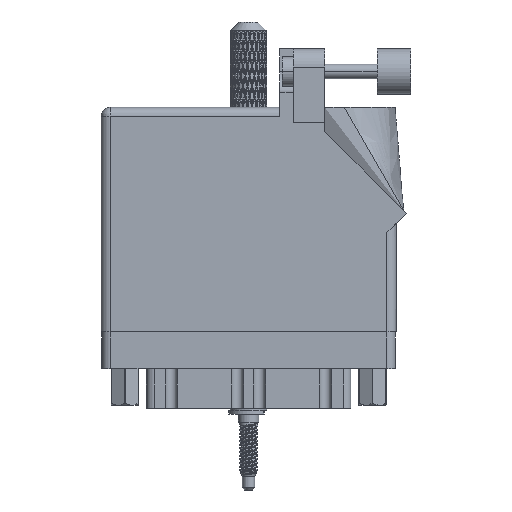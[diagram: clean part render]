
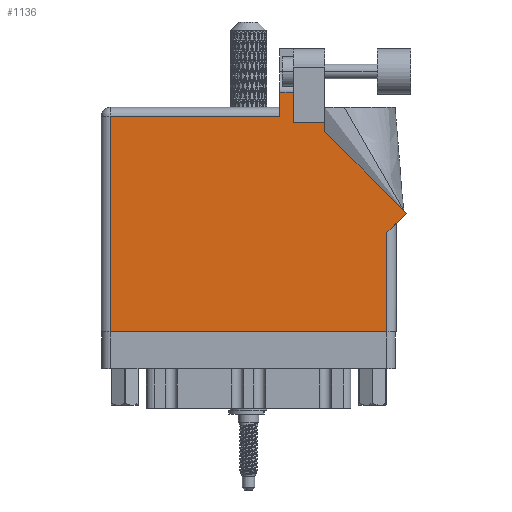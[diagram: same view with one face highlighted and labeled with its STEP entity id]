
A CAD part, front view. The second image highlights one B-rep face of the part: STEP entity #1136.
In plain terms, the highlighted face is planar.
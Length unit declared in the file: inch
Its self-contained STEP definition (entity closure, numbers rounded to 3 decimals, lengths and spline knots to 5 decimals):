
#1136 = ADVANCED_FACE ( 'NONE', ( #10595 ), #45646, .F. ) ;
#2997 = LINE ( 'NONE', #74816, #9502 ) ;
#4822 = LINE ( 'NONE', #14010, #57075 ) ;
#6854 = LINE ( 'NONE', #15484, #92922 ) ;
#8082 = VERTEX_POINT ( 'NONE', #25683 ) ;
#8295 = CARTESIAN_POINT ( 'NONE',  ( 1.948, 0., 0. ) ) ;
#8691 = VERTEX_POINT ( 'NONE', #42539 ) ;
#9327 = EDGE_CURVE ( 'NONE', #81317, #76900, #113542, .T. ) ;
#9394 = AXIS2_PLACEMENT_3D ( 'NONE', #80768, #61779, #37022 ) ;
#9502 = VECTOR ( 'NONE', #55290, 39.37008 ) ;
#9596 = ORIENTED_EDGE ( 'NONE', *, *, #113072, .T. ) ;
#10595 = FACE_OUTER_BOUND ( 'NONE', #31762, .T. ) ;
#11411 = EDGE_CURVE ( 'NONE', #18985, #8082, #17334, .T. ) ;
#14010 = CARTESIAN_POINT ( 'NONE',  ( 1.217, 1.53, 0. ) ) ;
#15283 = VECTOR ( 'NONE', #52614, 39.37008 ) ;
#15484 = CARTESIAN_POINT ( 'NONE',  ( 0., 1.468, 0. ) ) ;
#16804 = VECTOR ( 'NONE', #99911, 39.37008 ) ;
#17334 = LINE ( 'NONE', #52379, #65106 ) ;
#18728 = CARTESIAN_POINT ( 'NONE',  ( 2.08071, 0.80771, 0. ) ) ;
#18985 = VERTEX_POINT ( 'NONE', #39237 ) ;
#19264 = VECTOR ( 'NONE', #32398, 39.37008 ) ;
#20543 = CARTESIAN_POINT ( 'NONE',  ( 2.08071, 0.80771, 0. ) ) ;
#23062 = CARTESIAN_POINT ( 'NONE',  ( 1.311, 1.43, 0. ) ) ;
#23773 = VERTEX_POINT ( 'NONE', #82918 ) ;
#25299 = DIRECTION ( 'NONE',  ( 0., 1., 0. ) ) ;
#25683 = CARTESIAN_POINT ( 'NONE',  ( 1.311, 1.43, 0. ) ) ;
#27640 = VERTEX_POINT ( 'NONE', #107854 ) ;
#28287 = DIRECTION ( 'NONE',  ( 0., 1., 0. ) ) ;
#28886 = ORIENTED_EDGE ( 'NONE', *, *, #92803, .T. ) ;
#29039 = ORIENTED_EDGE ( 'NONE', *, *, #9327, .T. ) ;
#30234 = VECTOR ( 'NONE', #28287, 39.37008 ) ;
#31762 = EDGE_LOOP ( 'NONE', ( #52527, #9596, #28886, #35007, #96302, #73149, #81887, #29039, #71858, #47475, #35732 ) ) ;
#32072 = CARTESIAN_POINT ( 'NONE',  ( 1.217, 1.6315, 0. ) ) ;
#32131 = VERTEX_POINT ( 'NONE', #8295 ) ;
#32398 = DIRECTION ( 'NONE',  ( -0.707, 0.707, 0. ) ) ;
#34761 = DIRECTION ( 'NONE',  ( 0.707, 0.707, 0. ) ) ;
#34964 = EDGE_CURVE ( 'NONE', #32131, #81317, #70885, .T. ) ;
#35007 = ORIENTED_EDGE ( 'NONE', *, *, #108869, .T. ) ;
#35732 = ORIENTED_EDGE ( 'NONE', *, *, #11411, .T. ) ;
#37022 = DIRECTION ( 'NONE',  ( -1., 0., 0. ) ) ;
#39237 = CARTESIAN_POINT ( 'NONE',  ( 1.524, 1.43, 0. ) ) ;
#39376 = EDGE_CURVE ( 'NONE', #27640, #8691, #41122, .T. ) ;
#40375 = VECTOR ( 'NONE', #34761, 39.37008 ) ;
#40586 = VERTEX_POINT ( 'NONE', #61875 ) ;
#41122 = LINE ( 'NONE', #67587, #50276 ) ;
#42539 = CARTESIAN_POINT ( 'NONE',  ( 0.062, 0., 0. ) ) ;
#42853 = CARTESIAN_POINT ( 'NONE',  ( 2.01, 0.737, 0. ) ) ;
#43840 = EDGE_CURVE ( 'NONE', #23773, #18985, #87727, .T. ) ;
#45582 = CARTESIAN_POINT ( 'NONE',  ( 1.311, 1.6315, 0. ) ) ;
#45646 = PLANE ( 'NONE',  #9394 ) ;
#47475 = ORIENTED_EDGE ( 'NONE', *, *, #43840, .T. ) ;
#50276 = VECTOR ( 'NONE', #57240, 39.37008 ) ;
#50436 = VERTEX_POINT ( 'NONE', #32072 ) ;
#52379 = CARTESIAN_POINT ( 'NONE',  ( 1.524, 1.43, 0. ) ) ;
#52527 = ORIENTED_EDGE ( 'NONE', *, *, #66030, .T. ) ;
#52614 = DIRECTION ( 'NONE',  ( 0., 1., 0. ) ) ;
#52936 = DIRECTION ( 'NONE',  ( -1., 0., 0. ) ) ;
#53901 = VERTEX_POINT ( 'NONE', #45582 ) ;
#55290 = DIRECTION ( 'NONE',  ( 1., 0., 0. ) ) ;
#57075 = VECTOR ( 'NONE', #99722, 39.37008 ) ;
#57240 = DIRECTION ( 'NONE',  ( 0., -1., 0. ) ) ;
#61779 = DIRECTION ( 'NONE',  ( 0., 0., -1. ) ) ;
#61875 = CARTESIAN_POINT ( 'NONE',  ( 1.217, 1.468, 0. ) ) ;
#63960 = EDGE_CURVE ( 'NONE', #8691, #32131, #2997, .T. ) ;
#64825 = LINE ( 'NONE', #89596, #16804 ) ;
#65106 = VECTOR ( 'NONE', #52936, 39.37008 ) ;
#66030 = EDGE_CURVE ( 'NONE', #8082, #53901, #76524, .T. ) ;
#67258 = DIRECTION ( 'NONE',  ( -1., 0., 0. ) ) ;
#67587 = CARTESIAN_POINT ( 'NONE',  ( 0.062, 0., 0. ) ) ;
#68648 = CARTESIAN_POINT ( 'NONE',  ( 1.948, 0.675, 0. ) ) ;
#70885 = LINE ( 'NONE', #80649, #30234 ) ;
#71858 = ORIENTED_EDGE ( 'NONE', *, *, #87999, .T. ) ;
#73149 = ORIENTED_EDGE ( 'NONE', *, *, #63960, .T. ) ;
#73947 = VECTOR ( 'NONE', #25299, 39.37008 ) ;
#74816 = CARTESIAN_POINT ( 'NONE',  ( 0., 0., 0. ) ) ;
#76524 = LINE ( 'NONE', #23062, #73947 ) ;
#76900 = VERTEX_POINT ( 'NONE', #18728 ) ;
#79089 = CARTESIAN_POINT ( 'NONE',  ( 1.524, 1.36442, 0. ) ) ;
#80649 = CARTESIAN_POINT ( 'NONE',  ( 1.948, 0.737, 0. ) ) ;
#80768 = CARTESIAN_POINT ( 'NONE',  ( 0., 1.53, 0. ) ) ;
#81317 = VERTEX_POINT ( 'NONE', #68648 ) ;
#81887 = ORIENTED_EDGE ( 'NONE', *, *, #34964, .T. ) ;
#82918 = CARTESIAN_POINT ( 'NONE',  ( 1.524, 1.36442, 0. ) ) ;
#87727 = LINE ( 'NONE', #79089, #15283 ) ;
#87999 = EDGE_CURVE ( 'NONE', #76900, #23773, #111198, .T. ) ;
#89596 = CARTESIAN_POINT ( 'NONE',  ( 1.64177, 1.6315, 0. ) ) ;
#92803 = EDGE_CURVE ( 'NONE', #50436, #40586, #4822, .T. ) ;
#92922 = VECTOR ( 'NONE', #67258, 39.37008 ) ;
#96302 = ORIENTED_EDGE ( 'NONE', *, *, #39376, .T. ) ;
#99722 = DIRECTION ( 'NONE',  ( 0., -1., 0. ) ) ;
#99911 = DIRECTION ( 'NONE',  ( -1., 0., 0. ) ) ;
#107854 = CARTESIAN_POINT ( 'NONE',  ( 0.062, 1.468, 0. ) ) ;
#108869 = EDGE_CURVE ( 'NONE', #40586, #27640, #6854, .T. ) ;
#111198 = LINE ( 'NONE', #20543, #19264 ) ;
#113072 = EDGE_CURVE ( 'NONE', #53901, #50436, #64825, .T. ) ;
#113542 = LINE ( 'NONE', #42853, #40375 ) ;
